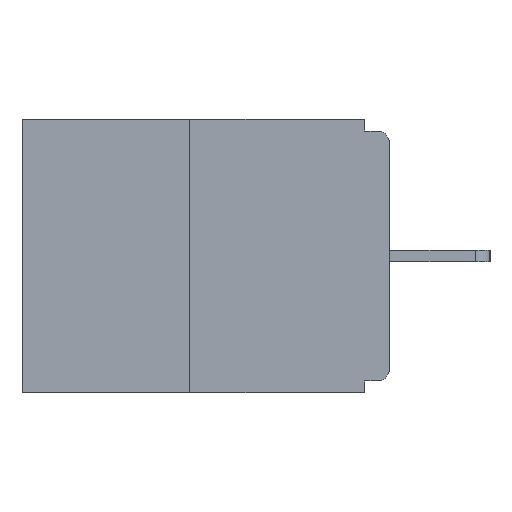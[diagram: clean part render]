
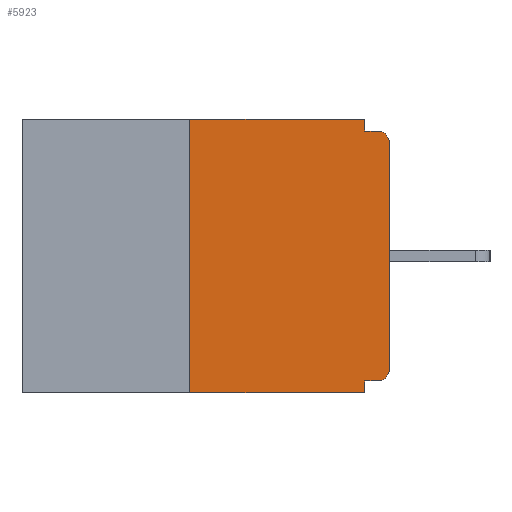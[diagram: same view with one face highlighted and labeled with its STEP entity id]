
A CAD part, left-side view. The second image highlights one B-rep face of the part: STEP entity #5923.
In plain terms, the highlighted planar face has unit normal (-1, 0, 0).
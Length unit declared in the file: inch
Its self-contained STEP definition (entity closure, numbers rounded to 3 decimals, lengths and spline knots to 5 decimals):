
#179 = EDGE_CURVE ( 'NONE', #5000, #11419, #7448, .T. ) ;
#586 = DIRECTION ( 'NONE',  ( 0., 0., -1. ) ) ;
#610 = ORIENTED_EDGE ( 'NONE', *, *, #4886, .F. ) ;
#1141 = EDGE_CURVE ( 'NONE', #5709, #11724, #15654, .T. ) ;
#1169 = CARTESIAN_POINT ( 'NONE',  ( 0., 0.25, 0. ) ) ;
#1196 = EDGE_CURVE ( 'NONE', #8899, #19507, #8281, .T. ) ;
#1203 = VECTOR ( 'NONE', #20624, 39.37008 ) ;
#1388 = VERTEX_POINT ( 'NONE', #16722 ) ;
#2086 = ORIENTED_EDGE ( 'NONE', *, *, #16766, .T. ) ;
#2102 = VERTEX_POINT ( 'NONE', #17768 ) ;
#2207 = CARTESIAN_POINT ( 'NONE',  ( 0., 0.25, 0. ) ) ;
#2676 = ORIENTED_EDGE ( 'NONE', *, *, #8580, .F. ) ;
#3123 = AXIS2_PLACEMENT_3D ( 'NONE', #9626, #20006, #18340 ) ;
#3397 = CARTESIAN_POINT ( 'NONE',  ( 0., 0.031, -0.343 ) ) ;
#3414 = ORIENTED_EDGE ( 'NONE', *, *, #1141, .T. ) ;
#3695 = AXIS2_PLACEMENT_3D ( 'NONE', #17402, #9016, #586 ) ;
#3867 = CARTESIAN_POINT ( 'NONE',  ( 0., 0., 0. ) ) ;
#4182 = ORIENTED_EDGE ( 'NONE', *, *, #4369, .F. ) ;
#4369 = EDGE_CURVE ( 'NONE', #5709, #5000, #14286, .T. ) ;
#4886 = EDGE_CURVE ( 'NONE', #13499, #11724, #17336, .T. ) ;
#5000 = VERTEX_POINT ( 'NONE', #1169 ) ;
#5138 = ORIENTED_EDGE ( 'NONE', *, *, #19752, .T. ) ;
#5288 = VECTOR ( 'NONE', #9091, 39.37008 ) ;
#5294 = VERTEX_POINT ( 'NONE', #14336 ) ;
#5504 = DIRECTION ( 'NONE',  ( 0., 0., -1. ) ) ;
#5709 = VERTEX_POINT ( 'NONE', #7537 ) ;
#5923 = ADVANCED_FACE ( 'NONE', ( #11514 ), #18236, .F. ) ;
#6255 = CARTESIAN_POINT ( 'NONE',  ( 0., 0., -0.03 ) ) ;
#7030 = VECTOR ( 'NONE', #21245, 39.37008 ) ;
#7170 = CARTESIAN_POINT ( 'NONE',  ( 0., 0.031, -0.343 ) ) ;
#7331 = DIRECTION ( 'NONE',  ( 0., -1., 0. ) ) ;
#7390 = ORIENTED_EDGE ( 'NONE', *, *, #8402, .F. ) ;
#7448 = LINE ( 'NONE', #14084, #19284 ) ;
#7537 = CARTESIAN_POINT ( 'NONE',  ( 0., 0.25, -0.343 ) ) ;
#7786 = VECTOR ( 'NONE', #9637, 39.37008 ) ;
#8256 = VECTOR ( 'NONE', #5504, 39.37008 ) ;
#8281 = CIRCLE ( 'NONE', #3695, 0.015 ) ;
#8402 = EDGE_CURVE ( 'NONE', #5294, #19507, #9305, .T. ) ;
#8580 = EDGE_CURVE ( 'NONE', #11419, #5294, #20017, .T. ) ;
#8751 = LINE ( 'NONE', #20476, #10422 ) ;
#8841 = DIRECTION ( 'NONE',  ( 0., 0., -1. ) ) ;
#8899 = VERTEX_POINT ( 'NONE', #6255 ) ;
#9016 = DIRECTION ( 'NONE',  ( -1., 0., 0. ) ) ;
#9091 = DIRECTION ( 'NONE',  ( 0., -1., 0. ) ) ;
#9305 = LINE ( 'NONE', #10867, #5288 ) ;
#9626 = CARTESIAN_POINT ( 'NONE',  ( 0., 0.015, -0.313 ) ) ;
#9637 = DIRECTION ( 'NONE',  ( 0., 0., -1. ) ) ;
#9738 = CARTESIAN_POINT ( 'NONE',  ( 0., 0.46, 0. ) ) ;
#10422 = VECTOR ( 'NONE', #12083, 39.37008 ) ;
#10867 = CARTESIAN_POINT ( 'NONE',  ( 0., 0., -0.015 ) ) ;
#11419 = VERTEX_POINT ( 'NONE', #11602 ) ;
#11514 = FACE_OUTER_BOUND ( 'NONE', #13121, .T. ) ;
#11600 = CIRCLE ( 'NONE', #3123, 0.015 ) ;
#11602 = CARTESIAN_POINT ( 'NONE',  ( 0., 0.031, 0. ) ) ;
#11724 = VERTEX_POINT ( 'NONE', #3397 ) ;
#12083 = DIRECTION ( 'NONE',  ( 0., 1., 0. ) ) ;
#12455 = CARTESIAN_POINT ( 'NONE',  ( 0., 0.46, -0.343 ) ) ;
#13121 = EDGE_LOOP ( 'NONE', ( #14713, #4182, #3414, #610, #18402, #5138, #2086, #13926, #7390, #2676 ) ) ;
#13499 = VERTEX_POINT ( 'NONE', #15461 ) ;
#13926 = ORIENTED_EDGE ( 'NONE', *, *, #1196, .T. ) ;
#14084 = CARTESIAN_POINT ( 'NONE',  ( 0., 0.46, 0. ) ) ;
#14286 = LINE ( 'NONE', #2207, #7030 ) ;
#14336 = CARTESIAN_POINT ( 'NONE',  ( 0., 0.031, -0.015 ) ) ;
#14610 = CARTESIAN_POINT ( 'NONE',  ( 0., 0.031, 0. ) ) ;
#14713 = ORIENTED_EDGE ( 'NONE', *, *, #179, .F. ) ;
#15461 = CARTESIAN_POINT ( 'NONE',  ( 0., 0.031, -0.328 ) ) ;
#15654 = LINE ( 'NONE', #12455, #1203 ) ;
#16024 = EDGE_CURVE ( 'NONE', #2102, #13499, #8751, .T. ) ;
#16471 = DIRECTION ( 'NONE',  ( 1., 0., 0. ) ) ;
#16722 = CARTESIAN_POINT ( 'NONE',  ( 0., 0., -0.313 ) ) ;
#16766 = EDGE_CURVE ( 'NONE', #1388, #8899, #20159, .T. ) ;
#17336 = LINE ( 'NONE', #7170, #8256 ) ;
#17402 = CARTESIAN_POINT ( 'NONE',  ( 0., 0.015, -0.03 ) ) ;
#17455 = DIRECTION ( 'NONE',  ( 0., 0., 1. ) ) ;
#17768 = CARTESIAN_POINT ( 'NONE',  ( 0., 0.015, -0.328 ) ) ;
#18236 = PLANE ( 'NONE',  #18329 ) ;
#18329 = AXIS2_PLACEMENT_3D ( 'NONE', #9738, #16471, #8841 ) ;
#18340 = DIRECTION ( 'NONE',  ( 0., 0., -1. ) ) ;
#18402 = ORIENTED_EDGE ( 'NONE', *, *, #16024, .F. ) ;
#19257 = VECTOR ( 'NONE', #17455, 39.37008 ) ;
#19284 = VECTOR ( 'NONE', #7331, 39.37008 ) ;
#19507 = VERTEX_POINT ( 'NONE', #20581 ) ;
#19752 = EDGE_CURVE ( 'NONE', #2102, #1388, #11600, .T. ) ;
#20006 = DIRECTION ( 'NONE',  ( -1., 0., 0. ) ) ;
#20017 = LINE ( 'NONE', #14610, #7786 ) ;
#20159 = LINE ( 'NONE', #3867, #19257 ) ;
#20476 = CARTESIAN_POINT ( 'NONE',  ( 0., 0., -0.328 ) ) ;
#20581 = CARTESIAN_POINT ( 'NONE',  ( 0., 0.015, -0.015 ) ) ;
#20624 = DIRECTION ( 'NONE',  ( 0., -1., 0. ) ) ;
#21245 = DIRECTION ( 'NONE',  ( 0., 0., 1. ) ) ;
